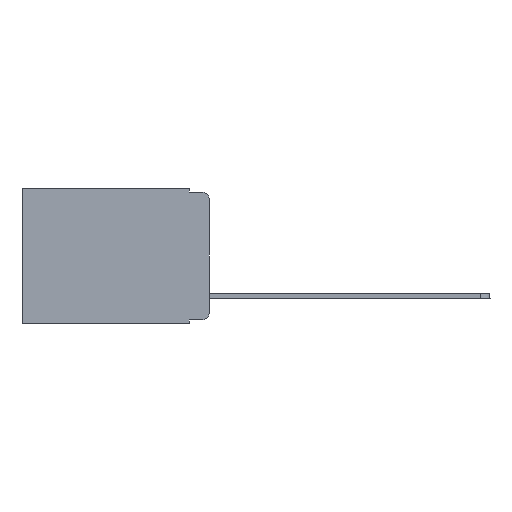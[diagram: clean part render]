
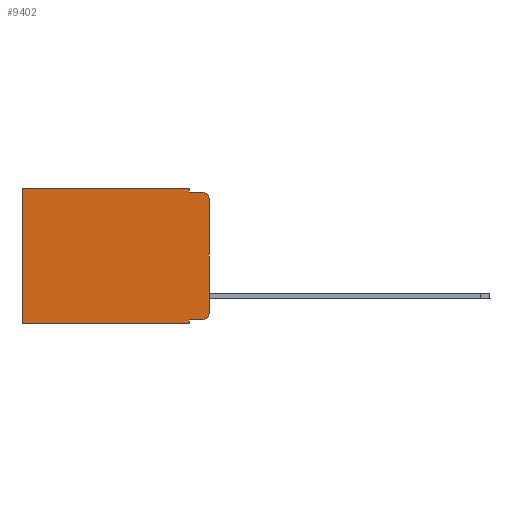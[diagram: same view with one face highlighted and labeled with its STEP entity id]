
A CAD part, left-side view. The second image highlights one B-rep face of the part: STEP entity #9402.
In plain terms, the highlighted planar face has unit normal (-1, 0, 0).
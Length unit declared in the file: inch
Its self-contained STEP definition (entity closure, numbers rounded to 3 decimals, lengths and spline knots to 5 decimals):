
#980 = DIRECTION ( 'NONE',  ( 0., 0., -1. ) ) ;
#1200 = VECTOR ( 'NONE', #8103, 39.37008 ) ;
#1232 = CARTESIAN_POINT ( 'NONE',  ( 0.298, 0.02, -0.03 ) ) ;
#2206 = LINE ( 'NONE', #13632, #8115 ) ;
#2260 = CARTESIAN_POINT ( 'NONE',  ( 0.298, 0.473, -0.343 ) ) ;
#2388 = VECTOR ( 'NONE', #7495, 39.37008 ) ;
#2417 = VECTOR ( 'NONE', #16510, 39.37008 ) ;
#2723 = CARTESIAN_POINT ( 'NONE',  ( 0.298, 0.051, -0.01 ) ) ;
#3106 = DIRECTION ( 'NONE',  ( 0., -1., 0. ) ) ;
#3236 = EDGE_CURVE ( 'NONE', #4425, #10803, #4937, .T. ) ;
#3942 = LINE ( 'NONE', #17025, #2388 ) ;
#4425 = VERTEX_POINT ( 'NONE', #9996 ) ;
#4619 = LINE ( 'NONE', #8391, #10702 ) ;
#4760 = AXIS2_PLACEMENT_3D ( 'NONE', #1232, #6745, #9430 ) ;
#4937 = LINE ( 'NONE', #6742, #1200 ) ;
#4939 = VERTEX_POINT ( 'NONE', #16806 ) ;
#5098 = CARTESIAN_POINT ( 'NONE',  ( 0.298, 0.02, -0.333 ) ) ;
#5882 = DIRECTION ( 'NONE',  ( 1., 0., 0. ) ) ;
#6130 = ORIENTED_EDGE ( 'NONE', *, *, #7420, .F. ) ;
#6361 = VECTOR ( 'NONE', #9421, 39.37008 ) ;
#6440 = VERTEX_POINT ( 'NONE', #13736 ) ;
#6575 = EDGE_CURVE ( 'NONE', #12281, #9913, #4619, .T. ) ;
#6742 = CARTESIAN_POINT ( 'NONE',  ( 0.298, 0.051, -0.333 ) ) ;
#6745 = DIRECTION ( 'NONE',  ( -1., 0., 0. ) ) ;
#6767 = ORIENTED_EDGE ( 'NONE', *, *, #14427, .T. ) ;
#7166 = DIRECTION ( 'NONE',  ( 0., 0., -1. ) ) ;
#7292 = ORIENTED_EDGE ( 'NONE', *, *, #6575, .T. ) ;
#7398 = DIRECTION ( 'NONE',  ( 0., 0., -1. ) ) ;
#7420 = EDGE_CURVE ( 'NONE', #12281, #16045, #10448, .T. ) ;
#7495 = DIRECTION ( 'NONE',  ( 0., 1., 0. ) ) ;
#7517 = EDGE_CURVE ( 'NONE', #16045, #4939, #10879, .T. ) ;
#7658 = ORIENTED_EDGE ( 'NONE', *, *, #16536, .T. ) ;
#7711 = VERTEX_POINT ( 'NONE', #2260 ) ;
#8086 = AXIS2_PLACEMENT_3D ( 'NONE', #12780, #5882, #7166 ) ;
#8103 = DIRECTION ( 'NONE',  ( 0., -1., 0. ) ) ;
#8107 = VERTEX_POINT ( 'NONE', #14430 ) ;
#8115 = VECTOR ( 'NONE', #980, 39.37008 ) ;
#8152 = AXIS2_PLACEMENT_3D ( 'NONE', #13988, #16717, #8395 ) ;
#8391 = CARTESIAN_POINT ( 'NONE',  ( 0.298, 0., 0. ) ) ;
#8395 = DIRECTION ( 'NONE',  ( 0., 0., -1. ) ) ;
#8752 = CIRCLE ( 'NONE', #8152, 0.02 ) ;
#9401 = CARTESIAN_POINT ( 'NONE',  ( 0.298, 0.051, 0. ) ) ;
#9402 = ADVANCED_FACE ( 'NONE', ( #11087 ), #10091, .F. ) ;
#9421 = DIRECTION ( 'NONE',  ( 0., 0., -1. ) ) ;
#9430 = DIRECTION ( 'NONE',  ( 0., 0., -1. ) ) ;
#9779 = VECTOR ( 'NONE', #7398, 39.37008 ) ;
#9913 = VERTEX_POINT ( 'NONE', #15235 ) ;
#9996 = CARTESIAN_POINT ( 'NONE',  ( 0.298, 0.051, -0.333 ) ) ;
#10062 = CARTESIAN_POINT ( 'NONE',  ( 0.298, 0.051, -0.01 ) ) ;
#10091 = PLANE ( 'NONE',  #8086 ) ;
#10448 = LINE ( 'NONE', #18034, #9779 ) ;
#10702 = VECTOR ( 'NONE', #11282, 39.37008 ) ;
#10761 = CARTESIAN_POINT ( 'NONE',  ( 0.298, 0.473, 0. ) ) ;
#10803 = VERTEX_POINT ( 'NONE', #5098 ) ;
#10830 = VERTEX_POINT ( 'NONE', #12240 ) ;
#10879 = LINE ( 'NONE', #10062, #15001 ) ;
#11087 = FACE_OUTER_BOUND ( 'NONE', #12081, .T. ) ;
#11093 = ORIENTED_EDGE ( 'NONE', *, *, #16882, .F. ) ;
#11282 = DIRECTION ( 'NONE',  ( 0., 1., 0. ) ) ;
#11410 = ORIENTED_EDGE ( 'NONE', *, *, #14404, .F. ) ;
#12078 = ORIENTED_EDGE ( 'NONE', *, *, #16674, .T. ) ;
#12081 = EDGE_LOOP ( 'NONE', ( #11410, #7658, #17241, #6130, #7292, #6767, #11093, #14715, #15099, #12078 ) ) ;
#12240 = CARTESIAN_POINT ( 'NONE',  ( 0.298, 0.051, -0.343 ) ) ;
#12281 = VERTEX_POINT ( 'NONE', #15178 ) ;
#12780 = CARTESIAN_POINT ( 'NONE',  ( 0.298, 0., 0. ) ) ;
#13632 = CARTESIAN_POINT ( 'NONE',  ( 0.298, 0., 0. ) ) ;
#13736 = CARTESIAN_POINT ( 'NONE',  ( 0.298, 0., -0.03 ) ) ;
#13988 = CARTESIAN_POINT ( 'NONE',  ( 0.298, 0.02, -0.313 ) ) ;
#13989 = EDGE_CURVE ( 'NONE', #4425, #10830, #15284, .T. ) ;
#14404 = EDGE_CURVE ( 'NONE', #6440, #8107, #2206, .T. ) ;
#14427 = EDGE_CURVE ( 'NONE', #9913, #7711, #14639, .T. ) ;
#14430 = CARTESIAN_POINT ( 'NONE',  ( 0.298, 0., -0.313 ) ) ;
#14639 = LINE ( 'NONE', #10761, #6361 ) ;
#14715 = ORIENTED_EDGE ( 'NONE', *, *, #13989, .F. ) ;
#14839 = CIRCLE ( 'NONE', #4760, 0.02 ) ;
#15001 = VECTOR ( 'NONE', #3106, 39.37008 ) ;
#15099 = ORIENTED_EDGE ( 'NONE', *, *, #3236, .T. ) ;
#15178 = CARTESIAN_POINT ( 'NONE',  ( 0.298, 0.051, 0. ) ) ;
#15235 = CARTESIAN_POINT ( 'NONE',  ( 0.298, 0.473, 0. ) ) ;
#15284 = LINE ( 'NONE', #9401, #2417 ) ;
#16045 = VERTEX_POINT ( 'NONE', #2723 ) ;
#16510 = DIRECTION ( 'NONE',  ( 0., 0., -1. ) ) ;
#16536 = EDGE_CURVE ( 'NONE', #6440, #4939, #14839, .T. ) ;
#16674 = EDGE_CURVE ( 'NONE', #10803, #8107, #8752, .T. ) ;
#16717 = DIRECTION ( 'NONE',  ( -1., 0., 0. ) ) ;
#16806 = CARTESIAN_POINT ( 'NONE',  ( 0.298, 0.02, -0.01 ) ) ;
#16882 = EDGE_CURVE ( 'NONE', #10830, #7711, #3942, .T. ) ;
#17025 = CARTESIAN_POINT ( 'NONE',  ( 0.298, 0., -0.343 ) ) ;
#17241 = ORIENTED_EDGE ( 'NONE', *, *, #7517, .F. ) ;
#18034 = CARTESIAN_POINT ( 'NONE',  ( 0.298, 0.051, 0. ) ) ;
